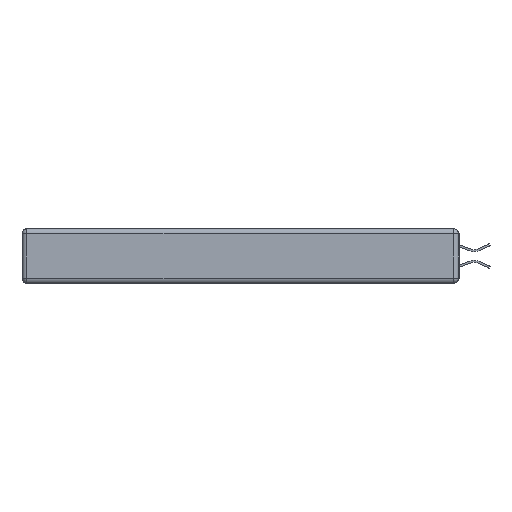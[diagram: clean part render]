
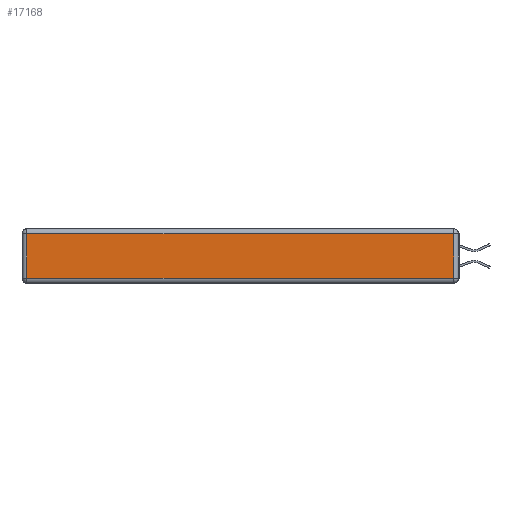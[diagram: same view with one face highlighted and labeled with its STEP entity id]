
A CAD part, left-side view. The second image highlights one B-rep face of the part: STEP entity #17168.
In plain terms, the highlighted planar face has unit normal (-1, 0, 0).
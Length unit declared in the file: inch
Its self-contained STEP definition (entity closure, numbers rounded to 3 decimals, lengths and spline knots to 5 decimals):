
#713 = LINE ( 'NONE', #4080, #22491 ) ;
#1263 = CARTESIAN_POINT ( 'NONE',  ( 0., 0.03, -0.03 ) ) ;
#1566 = CARTESIAN_POINT ( 'NONE',  ( 0., 0.03, -0.313 ) ) ;
#2429 = CARTESIAN_POINT ( 'NONE',  ( 0., 0.03, -0.343 ) ) ;
#3848 = CARTESIAN_POINT ( 'NONE',  ( 0., 2.75, -0.03 ) ) ;
#4049 = CARTESIAN_POINT ( 'NONE',  ( 0., 2.72, -0.03 ) ) ;
#4080 = CARTESIAN_POINT ( 'NONE',  ( 0., 0., -0.313 ) ) ;
#4687 = VERTEX_POINT ( 'NONE', #1566 ) ;
#5289 = DIRECTION ( 'NONE',  ( -1., 0., 0. ) ) ;
#6295 = VERTEX_POINT ( 'NONE', #1263 ) ;
#6357 = VERTEX_POINT ( 'NONE', #4049 ) ;
#6720 = CARTESIAN_POINT ( 'NONE',  ( 0., 2.72, -0.343 ) ) ;
#7331 = LINE ( 'NONE', #2429, #23842 ) ;
#7722 = EDGE_CURVE ( 'NONE', #6357, #27093, #15969, .T. ) ;
#8446 = ORIENTED_EDGE ( 'NONE', *, *, #7722, .T. ) ;
#8924 = EDGE_LOOP ( 'NONE', ( #13307, #13062, #12742, #8446 ) ) ;
#9371 = EDGE_CURVE ( 'NONE', #4687, #6295, #7331, .T. ) ;
#9813 = CARTESIAN_POINT ( 'NONE',  ( 0., 0., -0.343 ) ) ;
#10748 = VECTOR ( 'NONE', #26818, 39.37008 ) ;
#11578 = DIRECTION ( 'NONE',  ( 0., 0., 1. ) ) ;
#12742 = ORIENTED_EDGE ( 'NONE', *, *, #15704, .T. ) ;
#13052 = AXIS2_PLACEMENT_3D ( 'NONE', #9813, #5289, #11578 ) ;
#13062 = ORIENTED_EDGE ( 'NONE', *, *, #9371, .T. ) ;
#13307 = ORIENTED_EDGE ( 'NONE', *, *, #19762, .T. ) ;
#15639 = VECTOR ( 'NONE', #23601, 39.37008 ) ;
#15704 = EDGE_CURVE ( 'NONE', #6295, #6357, #16009, .T. ) ;
#15969 = LINE ( 'NONE', #6720, #15639 ) ;
#16009 = LINE ( 'NONE', #3848, #10748 ) ;
#17168 = ADVANCED_FACE ( 'NONE', ( #25161 ), #20415, .T. ) ;
#18848 = DIRECTION ( 'NONE',  ( 0., -1., 0. ) ) ;
#19762 = EDGE_CURVE ( 'NONE', #27093, #4687, #713, .T. ) ;
#20415 = PLANE ( 'NONE',  #13052 ) ;
#20659 = CARTESIAN_POINT ( 'NONE',  ( 0., 2.72, -0.313 ) ) ;
#22491 = VECTOR ( 'NONE', #18848, 39.37008 ) ;
#23601 = DIRECTION ( 'NONE',  ( 0., 0., -1. ) ) ;
#23842 = VECTOR ( 'NONE', #25870, 39.37008 ) ;
#25161 = FACE_OUTER_BOUND ( 'NONE', #8924, .T. ) ;
#25870 = DIRECTION ( 'NONE',  ( 0., 0., 1. ) ) ;
#26818 = DIRECTION ( 'NONE',  ( 0., 1., 0. ) ) ;
#27093 = VERTEX_POINT ( 'NONE', #20659 ) ;
